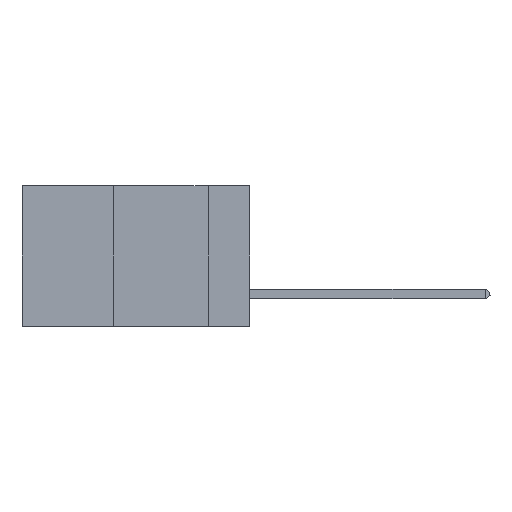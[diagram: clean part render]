
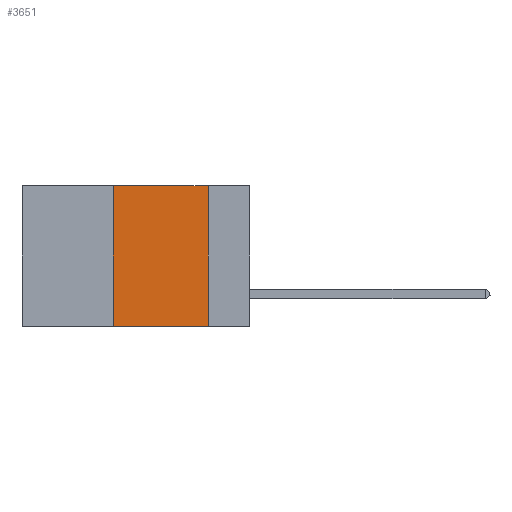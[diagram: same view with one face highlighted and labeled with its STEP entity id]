
A CAD part, left-side view. The second image highlights one B-rep face of the part: STEP entity #3651.
In plain terms, the highlighted planar face has unit normal (-1, 0, 0).
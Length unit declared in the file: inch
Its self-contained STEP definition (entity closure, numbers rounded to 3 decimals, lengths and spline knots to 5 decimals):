
#1340 = CARTESIAN_POINT ( 'NONE',  ( 0., 0.11, -0.37 ) ) ;
#1367 = ORIENTED_EDGE ( 'NONE', *, *, #1619, .T. ) ;
#1619 = EDGE_CURVE ( 'NONE', #10663, #3314, #2132, .T. ) ;
#2132 = LINE ( 'NONE', #13031, #14617 ) ;
#3314 = VERTEX_POINT ( 'NONE', #1340 ) ;
#3639 = DIRECTION ( 'NONE',  ( 0., 0., 1. ) ) ;
#3651 = ADVANCED_FACE ( 'NONE', ( #4905 ), #14841, .F. ) ;
#3946 = DIRECTION ( 'NONE',  ( 0., 0., -1. ) ) ;
#4905 = FACE_OUTER_BOUND ( 'NONE', #15178, .T. ) ;
#4953 = DIRECTION ( 'NONE',  ( 1., 0., 0. ) ) ;
#5315 = VECTOR ( 'NONE', #3639, 39.37008 ) ;
#5418 = VERTEX_POINT ( 'NONE', #13398 ) ;
#6845 = AXIS2_PLACEMENT_3D ( 'NONE', #9950, #4953, #3946 ) ;
#7241 = LINE ( 'NONE', #12091, #8007 ) ;
#7399 = EDGE_CURVE ( 'NONE', #5418, #7474, #13727, .T. ) ;
#7474 = VERTEX_POINT ( 'NONE', #14744 ) ;
#8007 = VECTOR ( 'NONE', #13321, 39.37008 ) ;
#8291 = DIRECTION ( 'NONE',  ( 0., -1., 0. ) ) ;
#8478 = CARTESIAN_POINT ( 'NONE',  ( 0., 0.36, 0. ) ) ;
#8496 = ORIENTED_EDGE ( 'NONE', *, *, #7399, .F. ) ;
#9164 = EDGE_CURVE ( 'NONE', #7474, #3314, #7241, .T. ) ;
#9950 = CARTESIAN_POINT ( 'NONE',  ( 0., 0.6, 0. ) ) ;
#10046 = ORIENTED_EDGE ( 'NONE', *, *, #9164, .F. ) ;
#10663 = VERTEX_POINT ( 'NONE', #14870 ) ;
#10746 = ORIENTED_EDGE ( 'NONE', *, *, #13222, .F. ) ;
#11253 = CARTESIAN_POINT ( 'NONE',  ( 0., 0.6, 0. ) ) ;
#11815 = VECTOR ( 'NONE', #13691, 39.37008 ) ;
#12091 = CARTESIAN_POINT ( 'NONE',  ( 0., 0.11, 0. ) ) ;
#12140 = LINE ( 'NONE', #8478, #5315 ) ;
#13031 = CARTESIAN_POINT ( 'NONE',  ( 0., 0.6, -0.37 ) ) ;
#13222 = EDGE_CURVE ( 'NONE', #10663, #5418, #12140, .T. ) ;
#13321 = DIRECTION ( 'NONE',  ( 0., 0., -1. ) ) ;
#13398 = CARTESIAN_POINT ( 'NONE',  ( 0., 0.36, 0. ) ) ;
#13691 = DIRECTION ( 'NONE',  ( 0., -1., 0. ) ) ;
#13727 = LINE ( 'NONE', #11253, #11815 ) ;
#14617 = VECTOR ( 'NONE', #8291, 39.37008 ) ;
#14744 = CARTESIAN_POINT ( 'NONE',  ( 0., 0.11, 0. ) ) ;
#14841 = PLANE ( 'NONE',  #6845 ) ;
#14870 = CARTESIAN_POINT ( 'NONE',  ( 0., 0.36, -0.37 ) ) ;
#15178 = EDGE_LOOP ( 'NONE', ( #10046, #8496, #10746, #1367 ) ) ;
